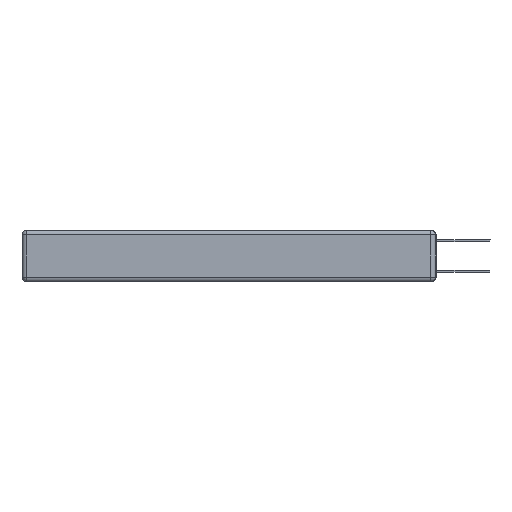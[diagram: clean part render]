
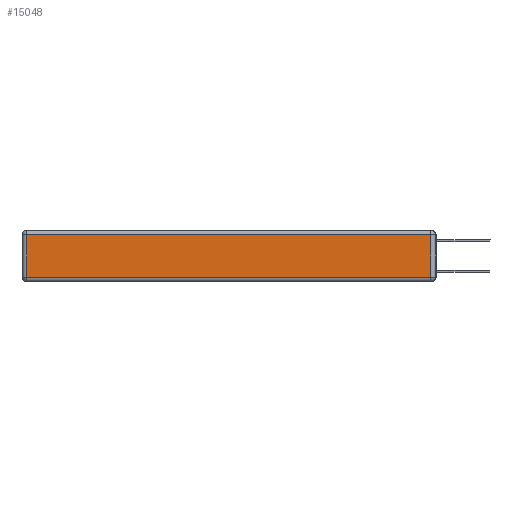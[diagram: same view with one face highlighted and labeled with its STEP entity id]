
A CAD part, left-side view. The second image highlights one B-rep face of the part: STEP entity #15048.
In plain terms, the highlighted planar face has unit normal (-1, 0, 0).
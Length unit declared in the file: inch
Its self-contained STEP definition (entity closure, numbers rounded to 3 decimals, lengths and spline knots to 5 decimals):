
#330 = ORIENTED_EDGE ( 'NONE', *, *, #2951, .T. ) ;
#659 = FACE_OUTER_BOUND ( 'NONE', #17166, .T. ) ;
#1319 = VERTEX_POINT ( 'NONE', #23864 ) ;
#2951 = EDGE_CURVE ( 'NONE', #1319, #24823, #20581, .T. ) ;
#4011 = ORIENTED_EDGE ( 'NONE', *, *, #10210, .T. ) ;
#4078 = CARTESIAN_POINT ( 'NONE',  ( 0., 0.03, -0.313 ) ) ;
#4083 = VERTEX_POINT ( 'NONE', #12575 ) ;
#4946 = DIRECTION ( 'NONE',  ( 0., -1., 0. ) ) ;
#5315 = CARTESIAN_POINT ( 'NONE',  ( 0., 2.72, -0.343 ) ) ;
#5378 = DIRECTION ( 'NONE',  ( 0., 0., 1. ) ) ;
#5562 = EDGE_CURVE ( 'NONE', #4083, #1319, #15148, .T. ) ;
#6070 = LINE ( 'NONE', #11739, #23739 ) ;
#7323 = EDGE_CURVE ( 'NONE', #24823, #18526, #22837, .T. ) ;
#7738 = DIRECTION ( 'NONE',  ( 0., 1., 0. ) ) ;
#8970 = ORIENTED_EDGE ( 'NONE', *, *, #7323, .T. ) ;
#10210 = EDGE_CURVE ( 'NONE', #18526, #4083, #6070, .T. ) ;
#11739 = CARTESIAN_POINT ( 'NONE',  ( 0., 2.75, -0.03 ) ) ;
#12565 = VECTOR ( 'NONE', #13194, 39.37008 ) ;
#12575 = CARTESIAN_POINT ( 'NONE',  ( 0., 2.72, -0.03 ) ) ;
#13194 = DIRECTION ( 'NONE',  ( 0., 0., -1. ) ) ;
#14937 = VECTOR ( 'NONE', #22973, 39.37008 ) ;
#15048 = ADVANCED_FACE ( 'NONE', ( #659 ), #24292, .T. ) ;
#15095 = DIRECTION ( 'NONE',  ( -1., 0., 0. ) ) ;
#15148 = LINE ( 'NONE', #5315, #12565 ) ;
#17166 = EDGE_LOOP ( 'NONE', ( #330, #8970, #4011, #23131 ) ) ;
#18526 = VERTEX_POINT ( 'NONE', #18587 ) ;
#18587 = CARTESIAN_POINT ( 'NONE',  ( 0., 0.03, -0.03 ) ) ;
#18712 = CARTESIAN_POINT ( 'NONE',  ( 0., 0., -0.343 ) ) ;
#20377 = AXIS2_PLACEMENT_3D ( 'NONE', #18712, #15095, #5378 ) ;
#20581 = LINE ( 'NONE', #22651, #21291 ) ;
#21291 = VECTOR ( 'NONE', #4946, 39.37008 ) ;
#22651 = CARTESIAN_POINT ( 'NONE',  ( 0., 0., -0.313 ) ) ;
#22837 = LINE ( 'NONE', #25269, #14937 ) ;
#22973 = DIRECTION ( 'NONE',  ( 0., 0., 1. ) ) ;
#23131 = ORIENTED_EDGE ( 'NONE', *, *, #5562, .T. ) ;
#23739 = VECTOR ( 'NONE', #7738, 39.37008 ) ;
#23864 = CARTESIAN_POINT ( 'NONE',  ( 0., 2.72, -0.313 ) ) ;
#24292 = PLANE ( 'NONE',  #20377 ) ;
#24823 = VERTEX_POINT ( 'NONE', #4078 ) ;
#25269 = CARTESIAN_POINT ( 'NONE',  ( 0., 0.03, -0.343 ) ) ;
